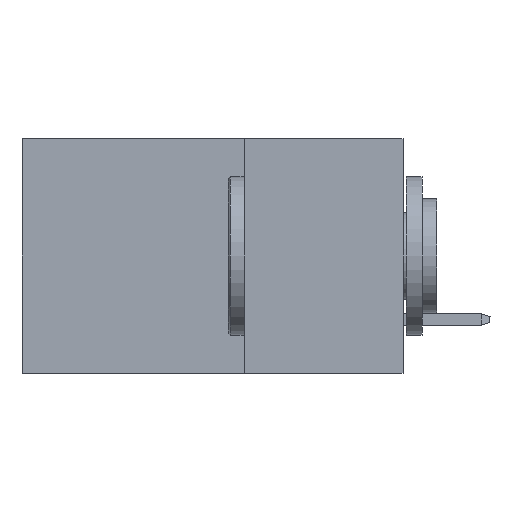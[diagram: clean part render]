
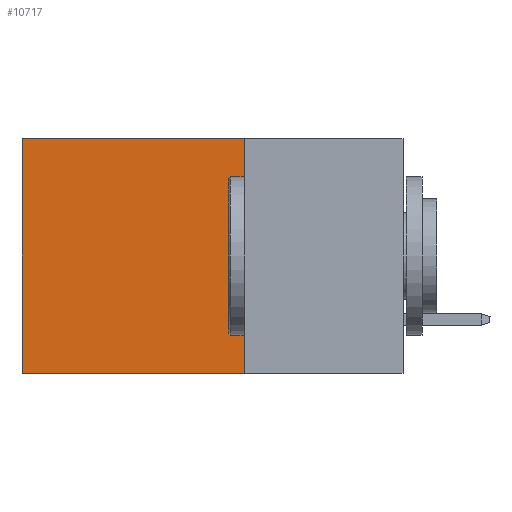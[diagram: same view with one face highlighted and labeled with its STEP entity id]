
A CAD part, left-side view. The second image highlights one B-rep face of the part: STEP entity #10717.
In plain terms, the highlighted planar face has unit normal (-1, 0, 0).
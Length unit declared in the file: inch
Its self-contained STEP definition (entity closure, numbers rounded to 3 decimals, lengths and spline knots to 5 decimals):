
#1446 = DIRECTION ( 'NONE',  ( 0., 0., -1. ) ) ;
#2295 = LINE ( 'NONE', #12714, #7310 ) ;
#3546 = CARTESIAN_POINT ( 'NONE',  ( 0.2875, 0.6, 0. ) ) ;
#3570 = EDGE_CURVE ( 'NONE', #25241, #27058, #2295, .T. ) ;
#3958 = ORIENTED_EDGE ( 'NONE', *, *, #3570, .T. ) ;
#7310 = VECTOR ( 'NONE', #31577, 39.37008 ) ;
#8518 = EDGE_CURVE ( 'NONE', #27058, #17613, #22369, .T. ) ;
#9096 = EDGE_CURVE ( 'NONE', #17795, #17613, #24007, .T. ) ;
#9804 = FACE_OUTER_BOUND ( 'NONE', #22785, .T. ) ;
#10717 = ADVANCED_FACE ( 'NONE', ( #9804 ), #25857, .F. ) ;
#11291 = CARTESIAN_POINT ( 'NONE',  ( 0.2875, 0.25, -0.37 ) ) ;
#12480 = CARTESIAN_POINT ( 'NONE',  ( 0.2875, 0.25, 0. ) ) ;
#12714 = CARTESIAN_POINT ( 'NONE',  ( 0.2875, 0.25, 0. ) ) ;
#12974 = VECTOR ( 'NONE', #17584, 39.37008 ) ;
#15553 = DIRECTION ( 'NONE',  ( 0., 1., 0. ) ) ;
#15628 = DIRECTION ( 'NONE',  ( 1., 0., 0. ) ) ;
#17584 = DIRECTION ( 'NONE',  ( 0., 0., -1. ) ) ;
#17586 = EDGE_CURVE ( 'NONE', #25241, #17795, #25593, .T. ) ;
#17613 = VERTEX_POINT ( 'NONE', #18361 ) ;
#17795 = VERTEX_POINT ( 'NONE', #11291 ) ;
#18014 = CARTESIAN_POINT ( 'NONE',  ( 0.2875, 0.25, 0. ) ) ;
#18101 = DIRECTION ( 'NONE',  ( 0., 0., -1. ) ) ;
#18107 = VECTOR ( 'NONE', #15553, 39.37008 ) ;
#18361 = CARTESIAN_POINT ( 'NONE',  ( 0.2875, 0.6, -0.37 ) ) ;
#20321 = VECTOR ( 'NONE', #1446, 39.37008 ) ;
#22369 = LINE ( 'NONE', #27976, #12974 ) ;
#22785 = EDGE_LOOP ( 'NONE', ( #32368, #33051, #27717, #3958 ) ) ;
#23466 = CARTESIAN_POINT ( 'NONE',  ( 0.2875, 0.25, 0. ) ) ;
#24007 = LINE ( 'NONE', #26636, #18107 ) ;
#25241 = VERTEX_POINT ( 'NONE', #23466 ) ;
#25593 = LINE ( 'NONE', #18014, #20321 ) ;
#25857 = PLANE ( 'NONE',  #31704 ) ;
#26636 = CARTESIAN_POINT ( 'NONE',  ( 0.2875, 0.25, -0.37 ) ) ;
#27058 = VERTEX_POINT ( 'NONE', #3546 ) ;
#27717 = ORIENTED_EDGE ( 'NONE', *, *, #17586, .F. ) ;
#27976 = CARTESIAN_POINT ( 'NONE',  ( 0.2875, 0.6, 0. ) ) ;
#31577 = DIRECTION ( 'NONE',  ( 0., 1., 0. ) ) ;
#31704 = AXIS2_PLACEMENT_3D ( 'NONE', #12480, #15628, #18101 ) ;
#32368 = ORIENTED_EDGE ( 'NONE', *, *, #8518, .T. ) ;
#33051 = ORIENTED_EDGE ( 'NONE', *, *, #9096, .F. ) ;
